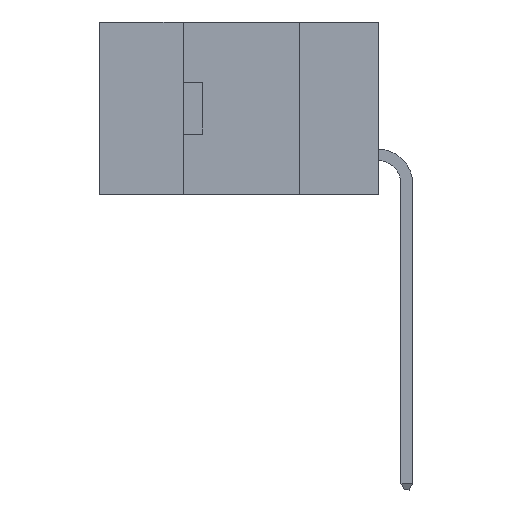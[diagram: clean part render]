
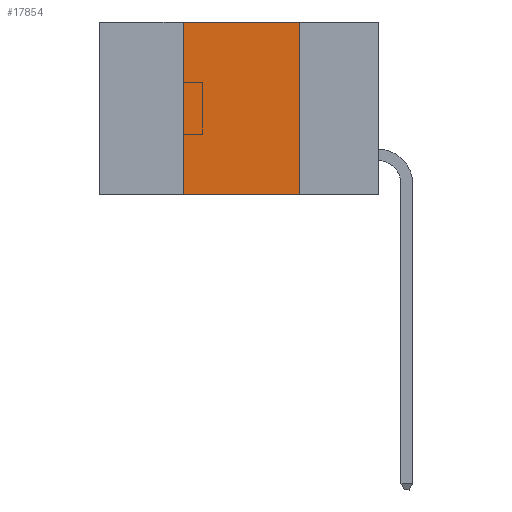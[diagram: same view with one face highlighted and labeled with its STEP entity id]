
A CAD part, left-side view. The second image highlights one B-rep face of the part: STEP entity #17854.
In plain terms, the highlighted planar face has unit normal (-1, 0, 0).
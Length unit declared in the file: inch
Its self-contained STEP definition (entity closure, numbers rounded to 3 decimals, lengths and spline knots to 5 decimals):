
#345 = ORIENTED_EDGE ( 'NONE', *, *, #21994, .F. ) ;
#2008 = DIRECTION ( 'NONE',  ( 0., -1., 0. ) ) ;
#2804 = CARTESIAN_POINT ( 'NONE',  ( 0., 0.17, 0. ) ) ;
#3465 = CARTESIAN_POINT ( 'NONE',  ( 0., 0.17, -0.37 ) ) ;
#4456 = DIRECTION ( 'NONE',  ( 0., 0., 1. ) ) ;
#5094 = VERTEX_POINT ( 'NONE', #13272 ) ;
#5453 = CARTESIAN_POINT ( 'NONE',  ( 0., 0.6, -0.37 ) ) ;
#5662 = AXIS2_PLACEMENT_3D ( 'NONE', #22193, #21916, #9947 ) ;
#5821 = EDGE_CURVE ( 'NONE', #5094, #19698, #6488, .T. ) ;
#6467 = VERTEX_POINT ( 'NONE', #3465 ) ;
#6488 = LINE ( 'NONE', #14689, #25968 ) ;
#9458 = EDGE_CURVE ( 'NONE', #5094, #6467, #11373, .T. ) ;
#9947 = DIRECTION ( 'NONE',  ( 0., 0., -1. ) ) ;
#11373 = LINE ( 'NONE', #5453, #21316 ) ;
#11677 = VECTOR ( 'NONE', #2008, 39.37008 ) ;
#11730 = CARTESIAN_POINT ( 'NONE',  ( 0., 0.17, -0.37 ) ) ;
#12249 = LINE ( 'NONE', #25021, #11677 ) ;
#12524 = VECTOR ( 'NONE', #15248, 39.37008 ) ;
#13272 = CARTESIAN_POINT ( 'NONE',  ( 0., 0.42, -0.37 ) ) ;
#14124 = FACE_OUTER_BOUND ( 'NONE', #18837, .T. ) ;
#14689 = CARTESIAN_POINT ( 'NONE',  ( 0., 0.42, -0.37 ) ) ;
#15248 = DIRECTION ( 'NONE',  ( 0., 0., -1. ) ) ;
#15285 = DIRECTION ( 'NONE',  ( 0., -1., 0. ) ) ;
#17110 = PLANE ( 'NONE',  #5662 ) ;
#17335 = EDGE_CURVE ( 'NONE', #22130, #6467, #21435, .T. ) ;
#17854 = ADVANCED_FACE ( 'NONE', ( #14124 ), #17110, .F. ) ;
#18837 = EDGE_LOOP ( 'NONE', ( #19140, #345, #22206, #21711 ) ) ;
#19140 = ORIENTED_EDGE ( 'NONE', *, *, #17335, .F. ) ;
#19698 = VERTEX_POINT ( 'NONE', #21456 ) ;
#21316 = VECTOR ( 'NONE', #15285, 39.37008 ) ;
#21435 = LINE ( 'NONE', #11730, #12524 ) ;
#21456 = CARTESIAN_POINT ( 'NONE',  ( 0., 0.42, 0. ) ) ;
#21711 = ORIENTED_EDGE ( 'NONE', *, *, #9458, .T. ) ;
#21916 = DIRECTION ( 'NONE',  ( 1., 0., 0. ) ) ;
#21994 = EDGE_CURVE ( 'NONE', #19698, #22130, #12249, .T. ) ;
#22130 = VERTEX_POINT ( 'NONE', #2804 ) ;
#22193 = CARTESIAN_POINT ( 'NONE',  ( 0., 0.6, 0. ) ) ;
#22206 = ORIENTED_EDGE ( 'NONE', *, *, #5821, .F. ) ;
#25021 = CARTESIAN_POINT ( 'NONE',  ( 0., 0.6, 0. ) ) ;
#25968 = VECTOR ( 'NONE', #4456, 39.37008 ) ;
